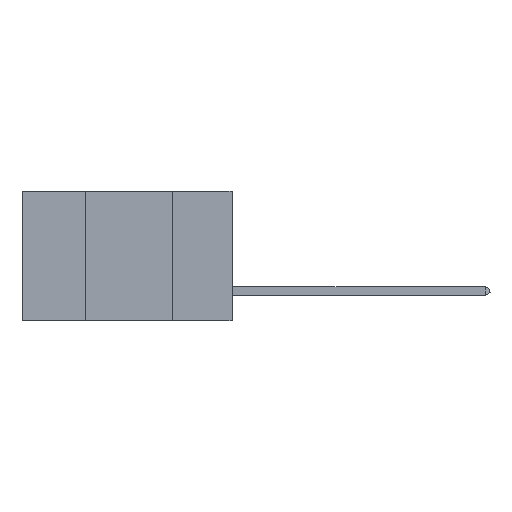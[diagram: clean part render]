
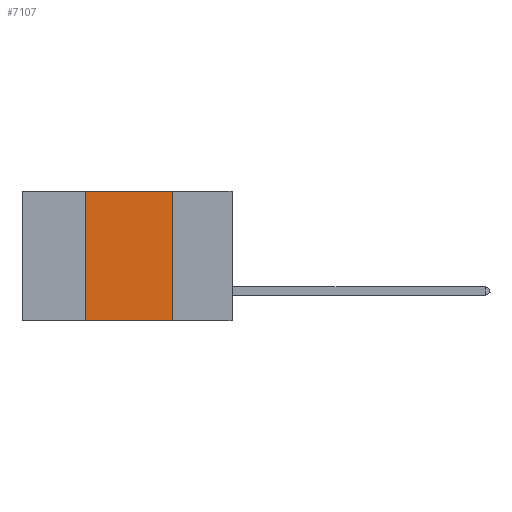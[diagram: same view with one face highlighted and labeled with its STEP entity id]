
A CAD part, left-side view. The second image highlights one B-rep face of the part: STEP entity #7107.
In plain terms, the highlighted planar face has unit normal (-1, 0, 0).
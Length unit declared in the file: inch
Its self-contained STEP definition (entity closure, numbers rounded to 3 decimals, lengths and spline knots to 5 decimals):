
#283 = ORIENTED_EDGE ( 'NONE', *, *, #6862, .F. ) ;
#1084 = VERTEX_POINT ( 'NONE', #7028 ) ;
#1714 = FACE_OUTER_BOUND ( 'NONE', #11622, .T. ) ;
#1814 = CARTESIAN_POINT ( 'NONE',  ( 0., 0.6, 0. ) ) ;
#3289 = LINE ( 'NONE', #14327, #4523 ) ;
#3542 = VERTEX_POINT ( 'NONE', #7830 ) ;
#3934 = DIRECTION ( 'NONE',  ( 1., 0., 0. ) ) ;
#4007 = CARTESIAN_POINT ( 'NONE',  ( 0., 0.42, 0. ) ) ;
#4523 = VECTOR ( 'NONE', #14132, 39.37008 ) ;
#4739 = ORIENTED_EDGE ( 'NONE', *, *, #4784, .T. ) ;
#4741 = CARTESIAN_POINT ( 'NONE',  ( 0., 0.6, 0. ) ) ;
#4784 = EDGE_CURVE ( 'NONE', #3542, #10517, #11287, .T. ) ;
#5125 = DIRECTION ( 'NONE',  ( 0., -1., 0. ) ) ;
#5462 = EDGE_CURVE ( 'NONE', #1084, #14155, #11451, .T. ) ;
#5658 = DIRECTION ( 'NONE',  ( 0., -1., 0. ) ) ;
#6172 = VECTOR ( 'NONE', #14475, 39.37008 ) ;
#6862 = EDGE_CURVE ( 'NONE', #3542, #1084, #14456, .T. ) ;
#6924 = VECTOR ( 'NONE', #5125, 39.37008 ) ;
#7012 = PLANE ( 'NONE',  #12056 ) ;
#7028 = CARTESIAN_POINT ( 'NONE',  ( 0., 0.42, 0. ) ) ;
#7107 = ADVANCED_FACE ( 'NONE', ( #1714 ), #7012, .F. ) ;
#7573 = EDGE_CURVE ( 'NONE', #14155, #10517, #3289, .T. ) ;
#7806 = CARTESIAN_POINT ( 'NONE',  ( 0., 0.17, 0. ) ) ;
#7830 = CARTESIAN_POINT ( 'NONE',  ( 0., 0.42, -0.37 ) ) ;
#8030 = VECTOR ( 'NONE', #5658, 39.37008 ) ;
#8060 = CARTESIAN_POINT ( 'NONE',  ( 0., 0.6, -0.37 ) ) ;
#8554 = DIRECTION ( 'NONE',  ( 0., 0., -1. ) ) ;
#10517 = VERTEX_POINT ( 'NONE', #13079 ) ;
#11221 = ORIENTED_EDGE ( 'NONE', *, *, #7573, .F. ) ;
#11287 = LINE ( 'NONE', #8060, #8030 ) ;
#11451 = LINE ( 'NONE', #1814, #6924 ) ;
#11622 = EDGE_LOOP ( 'NONE', ( #11221, #12990, #283, #4739 ) ) ;
#12056 = AXIS2_PLACEMENT_3D ( 'NONE', #4741, #3934, #8554 ) ;
#12990 = ORIENTED_EDGE ( 'NONE', *, *, #5462, .F. ) ;
#13079 = CARTESIAN_POINT ( 'NONE',  ( 0., 0.17, -0.37 ) ) ;
#14132 = DIRECTION ( 'NONE',  ( 0., 0., -1. ) ) ;
#14155 = VERTEX_POINT ( 'NONE', #7806 ) ;
#14327 = CARTESIAN_POINT ( 'NONE',  ( 0., 0.17, 0. ) ) ;
#14456 = LINE ( 'NONE', #4007, #6172 ) ;
#14475 = DIRECTION ( 'NONE',  ( 0., 0., 1. ) ) ;
